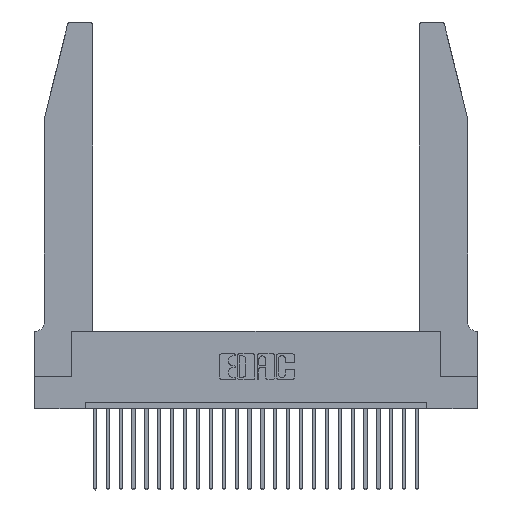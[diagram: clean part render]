
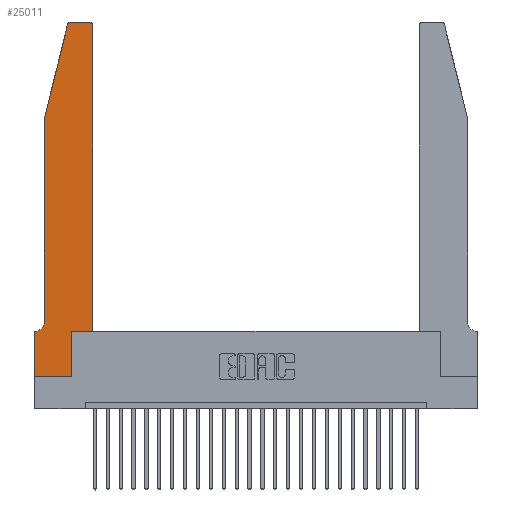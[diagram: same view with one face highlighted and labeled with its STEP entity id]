
A CAD part, top view. The second image highlights one B-rep face of the part: STEP entity #25011.
In plain terms, the highlighted planar face has unit normal (0, 0, 1).
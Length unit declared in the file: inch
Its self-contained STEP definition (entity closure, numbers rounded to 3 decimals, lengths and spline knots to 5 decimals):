
#34 = VERTEX_POINT ( 'NONE', #7694 ) ;
#213 = ORIENTED_EDGE ( 'NONE', *, *, #19313, .T. ) ;
#460 = VECTOR ( 'NONE', #1690, 39.37008 ) ;
#1128 = DIRECTION ( 'NONE',  ( 1., 0., 0. ) ) ;
#1134 = VERTEX_POINT ( 'NONE', #18221 ) ;
#1183 = DIRECTION ( 'NONE',  ( 0., 0., 1. ) ) ;
#1286 = VERTEX_POINT ( 'NONE', #2868 ) ;
#1394 = ORIENTED_EDGE ( 'NONE', *, *, #19591, .T. ) ;
#1690 = DIRECTION ( 'NONE',  ( -1., 0., 0. ) ) ;
#1693 = LINE ( 'NONE', #7208, #4568 ) ;
#1806 = CARTESIAN_POINT ( 'NONE',  ( 0.284, 2.75, 0.37 ) ) ;
#2868 = CARTESIAN_POINT ( 'NONE',  ( 0., 0., 0.37 ) ) ;
#2941 = CARTESIAN_POINT ( 'NONE',  ( 0.2865, 0., 0.37 ) ) ;
#3131 = DIRECTION ( 'NONE',  ( 0., -1., 0. ) ) ;
#3205 = CIRCLE ( 'NONE', #21497, 0.03 ) ;
#3233 = DIRECTION ( 'NONE',  ( 0., 0., 1. ) ) ;
#3272 = ORIENTED_EDGE ( 'NONE', *, *, #17169, .T. ) ;
#3479 = DIRECTION ( 'NONE',  ( 0., 1., 0. ) ) ;
#3783 = VERTEX_POINT ( 'NONE', #10227 ) ;
#3785 = CARTESIAN_POINT ( 'NONE',  ( 0., 0.35, 0.37 ) ) ;
#4109 = ORIENTED_EDGE ( 'NONE', *, *, #21237, .T. ) ;
#4402 = LINE ( 'NONE', #9323, #10504 ) ;
#4568 = VECTOR ( 'NONE', #1128, 39.37008 ) ;
#4624 = DIRECTION ( 'NONE',  ( 1., 0., 0. ) ) ;
#5061 = CARTESIAN_POINT ( 'NONE',  ( 0.4505, 0.35, 0.37 ) ) ;
#5297 = AXIS2_PLACEMENT_3D ( 'NONE', #11762, #3233, #11494 ) ;
#5517 = VECTOR ( 'NONE', #15108, 39.37008 ) ;
#5594 = LINE ( 'NONE', #10158, #14579 ) ;
#5872 = VERTEX_POINT ( 'NONE', #23113 ) ;
#6071 = DIRECTION ( 'NONE',  ( 0., 0., 1. ) ) ;
#6335 = LINE ( 'NONE', #25832, #12424 ) ;
#6627 = ORIENTED_EDGE ( 'NONE', *, *, #24446, .T. ) ;
#6676 = ORIENTED_EDGE ( 'NONE', *, *, #22275, .T. ) ;
#6864 = CARTESIAN_POINT ( 'NONE',  ( 0.0755, 2., 0.37 ) ) ;
#6885 = EDGE_CURVE ( 'NONE', #17871, #23748, #20263, .T. ) ;
#6932 = CARTESIAN_POINT ( 'NONE',  ( 0.4505, 2.72, 0.37 ) ) ;
#7208 = CARTESIAN_POINT ( 'NONE',  ( 0., 0., 0.37 ) ) ;
#7281 = CIRCLE ( 'NONE', #16060, 0.03 ) ;
#7399 = VECTOR ( 'NONE', #20912, 39.37008 ) ;
#7694 = CARTESIAN_POINT ( 'NONE',  ( 0.25487, 2.72718, 0.37 ) ) ;
#8902 = AXIS2_PLACEMENT_3D ( 'NONE', #22688, #12683, #20733 ) ;
#9323 = CARTESIAN_POINT ( 'NONE',  ( 0.0755, 2., 0.37 ) ) ;
#9535 = EDGE_CURVE ( 'NONE', #15329, #3783, #4402, .T. ) ;
#9863 = ORIENTED_EDGE ( 'NONE', *, *, #22858, .T. ) ;
#10158 = CARTESIAN_POINT ( 'NONE',  ( 0.4505, 0.35, 0.37 ) ) ;
#10188 = VERTEX_POINT ( 'NONE', #17294 ) ;
#10227 = CARTESIAN_POINT ( 'NONE',  ( 0.0755, 0.42, 0.37 ) ) ;
#10366 = VERTEX_POINT ( 'NONE', #3785 ) ;
#10504 = VECTOR ( 'NONE', #21733, 39.37008 ) ;
#10607 = CARTESIAN_POINT ( 'NONE',  ( 0.284, 2.72, 0.37 ) ) ;
#11162 = FACE_OUTER_BOUND ( 'NONE', #13343, .T. ) ;
#11494 = DIRECTION ( 'NONE',  ( 1., 0., 0. ) ) ;
#11762 = CARTESIAN_POINT ( 'NONE',  ( 0., 0.35, 0.37 ) ) ;
#11854 = CIRCLE ( 'NONE', #8902, 0.07 ) ;
#12170 = VECTOR ( 'NONE', #3131, 39.37008 ) ;
#12424 = VECTOR ( 'NONE', #3479, 39.37008 ) ;
#12683 = DIRECTION ( 'NONE',  ( 0., 0., -1. ) ) ;
#13343 = EDGE_LOOP ( 'NONE', ( #6676, #213, #1394, #18605, #26441, #9863, #6627, #3272, #18379, #24409, #16131, #4109 ) ) ;
#13414 = VERTEX_POINT ( 'NONE', #1806 ) ;
#13636 = PLANE ( 'NONE',  #5297 ) ;
#14235 = CARTESIAN_POINT ( 'NONE',  ( 0.0755, 0.35, 0.37 ) ) ;
#14269 = DIRECTION ( 'NONE',  ( 1., 0., 0. ) ) ;
#14579 = VECTOR ( 'NONE', #14269, 39.37008 ) ;
#15061 = LINE ( 'NONE', #20826, #7399 ) ;
#15108 = DIRECTION ( 'NONE',  ( 0., 1., 0. ) ) ;
#15329 = VERTEX_POINT ( 'NONE', #6864 ) ;
#15873 = CARTESIAN_POINT ( 'NONE',  ( 0.2605, 2.75, 0.37 ) ) ;
#15883 = VECTOR ( 'NONE', #22138, 39.37008 ) ;
#15919 = CARTESIAN_POINT ( 'NONE',  ( 0.4205, 2.72, 0.37 ) ) ;
#16060 = AXIS2_PLACEMENT_3D ( 'NONE', #15919, #6071, #20238 ) ;
#16131 = ORIENTED_EDGE ( 'NONE', *, *, #6885, .T. ) ;
#17169 = EDGE_CURVE ( 'NONE', #1286, #17716, #1693, .T. ) ;
#17294 = CARTESIAN_POINT ( 'NONE',  ( 0.4205, 2.75, 0.37 ) ) ;
#17617 = LINE ( 'NONE', #21842, #12170 ) ;
#17653 = CARTESIAN_POINT ( 'NONE',  ( 0.4505, 0.35, 0.37 ) ) ;
#17716 = VERTEX_POINT ( 'NONE', #2941 ) ;
#17871 = VERTEX_POINT ( 'NONE', #17653 ) ;
#18221 = CARTESIAN_POINT ( 'NONE',  ( 0.2865, 0.35, 0.37 ) ) ;
#18379 = ORIENTED_EDGE ( 'NONE', *, *, #21108, .T. ) ;
#18605 = ORIENTED_EDGE ( 'NONE', *, *, #9535, .T. ) ;
#19313 = EDGE_CURVE ( 'NONE', #13414, #34, #3205, .T. ) ;
#19591 = EDGE_CURVE ( 'NONE', #34, #15329, #15061, .T. ) ;
#20238 = DIRECTION ( 'NONE',  ( 1., 0., 0. ) ) ;
#20263 = LINE ( 'NONE', #5061, #5517 ) ;
#20733 = DIRECTION ( 'NONE',  ( -1., 0., 0. ) ) ;
#20826 = CARTESIAN_POINT ( 'NONE',  ( 0.0755, 2., 0.37 ) ) ;
#20912 = DIRECTION ( 'NONE',  ( -0.239, -0.971, 0. ) ) ;
#21108 = EDGE_CURVE ( 'NONE', #17716, #1134, #6335, .T. ) ;
#21237 = EDGE_CURVE ( 'NONE', #23748, #10188, #7281, .T. ) ;
#21497 = AXIS2_PLACEMENT_3D ( 'NONE', #10607, #1183, #4624 ) ;
#21733 = DIRECTION ( 'NONE',  ( 0., -1., 0. ) ) ;
#21842 = CARTESIAN_POINT ( 'NONE',  ( 0., 0., 0.37 ) ) ;
#22138 = DIRECTION ( 'NONE',  ( -1., 0., 0. ) ) ;
#22275 = EDGE_CURVE ( 'NONE', #10188, #13414, #22607, .T. ) ;
#22411 = EDGE_CURVE ( 'NONE', #1134, #17871, #5594, .T. ) ;
#22607 = LINE ( 'NONE', #15873, #15883 ) ;
#22688 = CARTESIAN_POINT ( 'NONE',  ( 0.0055, 0.42, 0.37 ) ) ;
#22858 = EDGE_CURVE ( 'NONE', #5872, #10366, #22865, .T. ) ;
#22865 = LINE ( 'NONE', #14235, #460 ) ;
#23113 = CARTESIAN_POINT ( 'NONE',  ( 0.0055, 0.35, 0.37 ) ) ;
#23548 = EDGE_CURVE ( 'NONE', #3783, #5872, #11854, .T. ) ;
#23748 = VERTEX_POINT ( 'NONE', #6932 ) ;
#24409 = ORIENTED_EDGE ( 'NONE', *, *, #22411, .T. ) ;
#24446 = EDGE_CURVE ( 'NONE', #10366, #1286, #17617, .T. ) ;
#25011 = ADVANCED_FACE ( 'NONE', ( #11162 ), #13636, .T. ) ;
#25832 = CARTESIAN_POINT ( 'NONE',  ( 0.2865, 0.35, 0.37 ) ) ;
#26441 = ORIENTED_EDGE ( 'NONE', *, *, #23548, .T. ) ;
